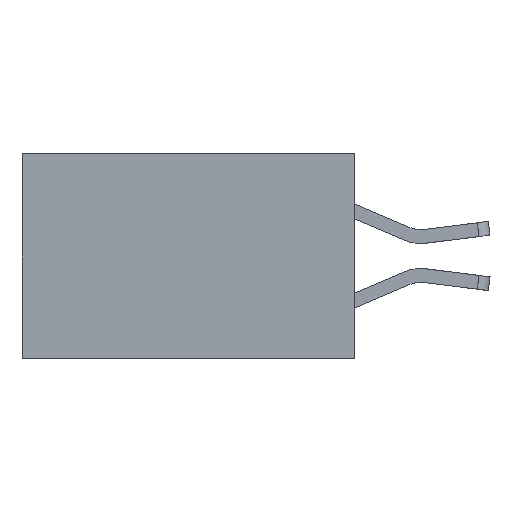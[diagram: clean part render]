
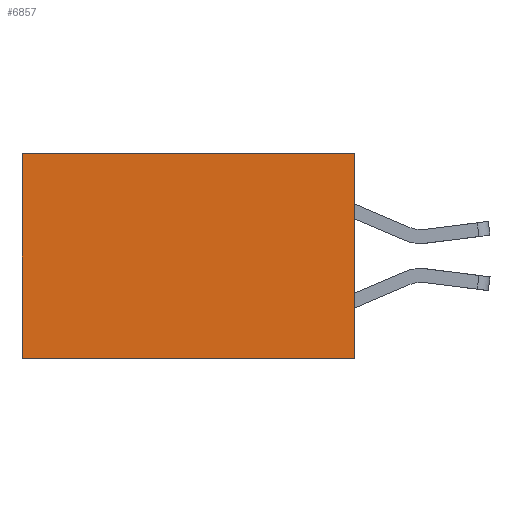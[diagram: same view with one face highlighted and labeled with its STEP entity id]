
A CAD part, left-side view. The second image highlights one B-rep face of the part: STEP entity #6857.
In plain terms, the highlighted planar face has unit normal (-1, 0, 0).
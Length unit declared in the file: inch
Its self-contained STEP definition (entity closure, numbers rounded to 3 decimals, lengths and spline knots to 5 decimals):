
#616 = CARTESIAN_POINT ( 'NONE',  ( 0.2615, 0., 0. ) ) ;
#975 = CARTESIAN_POINT ( 'NONE',  ( 0.2615, 0.6, -0.37 ) ) ;
#978 = VERTEX_POINT ( 'NONE', #975 ) ;
#1176 = VECTOR ( 'NONE', #5200, 39.37008 ) ;
#1644 = VECTOR ( 'NONE', #5336, 39.37008 ) ;
#2407 = EDGE_CURVE ( 'NONE', #3262, #978, #3745, .T. ) ;
#2762 = VECTOR ( 'NONE', #5732, 39.37008 ) ;
#2813 = PLANE ( 'NONE',  #5994 ) ;
#3152 = LINE ( 'NONE', #8246, #1176 ) ;
#3157 = EDGE_CURVE ( 'NONE', #7880, #3262, #3613, .T. ) ;
#3262 = VERTEX_POINT ( 'NONE', #4843 ) ;
#3471 = VERTEX_POINT ( 'NONE', #4491 ) ;
#3613 = LINE ( 'NONE', #3882, #1644 ) ;
#3745 = LINE ( 'NONE', #4620, #7671 ) ;
#3882 = CARTESIAN_POINT ( 'NONE',  ( 0.2615, 0., 0. ) ) ;
#4292 = DIRECTION ( 'NONE',  ( 1., 0., 0. ) ) ;
#4491 = CARTESIAN_POINT ( 'NONE',  ( 0.2615, 0., -0.37 ) ) ;
#4620 = CARTESIAN_POINT ( 'NONE',  ( 0.2615, 0.6, -0.37 ) ) ;
#4645 = DIRECTION ( 'NONE',  ( 0., 0., -1. ) ) ;
#4843 = CARTESIAN_POINT ( 'NONE',  ( 0.2615, 0.6, 0. ) ) ;
#5000 = CARTESIAN_POINT ( 'NONE',  ( 0.2615, 0., -0.37 ) ) ;
#5200 = DIRECTION ( 'NONE',  ( 0., 0., -1. ) ) ;
#5305 = ORIENTED_EDGE ( 'NONE', *, *, #3157, .T. ) ;
#5310 = FACE_OUTER_BOUND ( 'NONE', #6628, .T. ) ;
#5336 = DIRECTION ( 'NONE',  ( 0., 1., 0. ) ) ;
#5652 = EDGE_CURVE ( 'NONE', #3471, #978, #8439, .T. ) ;
#5732 = DIRECTION ( 'NONE',  ( 0., 1., 0. ) ) ;
#5994 = AXIS2_PLACEMENT_3D ( 'NONE', #8755, #4292, #9445 ) ;
#6628 = EDGE_LOOP ( 'NONE', ( #7916, #8288, #8380, #5305 ) ) ;
#6857 = ADVANCED_FACE ( 'NONE', ( #5310 ), #2813, .F. ) ;
#7671 = VECTOR ( 'NONE', #4645, 39.37008 ) ;
#7880 = VERTEX_POINT ( 'NONE', #616 ) ;
#7916 = ORIENTED_EDGE ( 'NONE', *, *, #2407, .T. ) ;
#8246 = CARTESIAN_POINT ( 'NONE',  ( 0.2615, 0., -0.37 ) ) ;
#8288 = ORIENTED_EDGE ( 'NONE', *, *, #5652, .F. ) ;
#8380 = ORIENTED_EDGE ( 'NONE', *, *, #9336, .F. ) ;
#8439 = LINE ( 'NONE', #5000, #2762 ) ;
#8755 = CARTESIAN_POINT ( 'NONE',  ( 0.2615, 0., -0.37 ) ) ;
#9336 = EDGE_CURVE ( 'NONE', #7880, #3471, #3152, .T. ) ;
#9445 = DIRECTION ( 'NONE',  ( 0., 0., -1. ) ) ;
